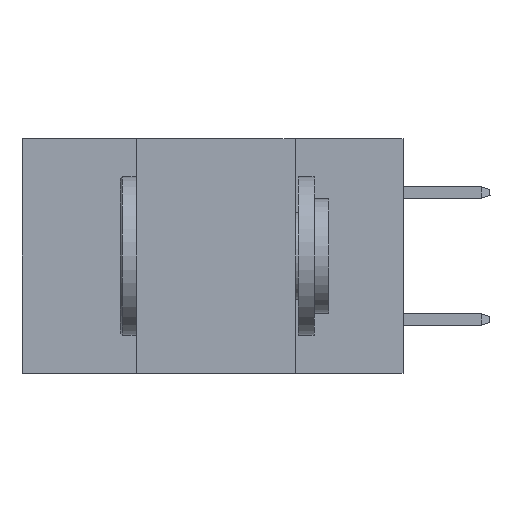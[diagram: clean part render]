
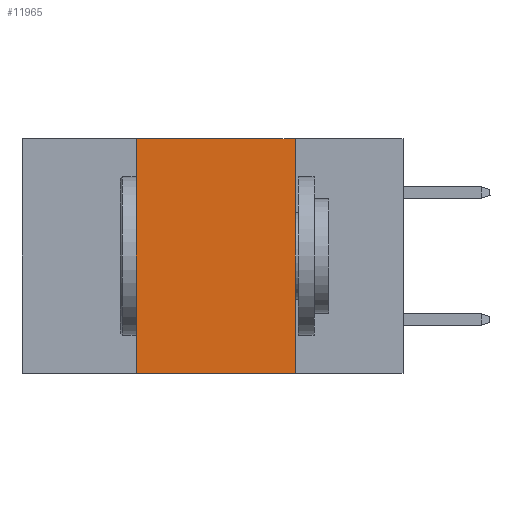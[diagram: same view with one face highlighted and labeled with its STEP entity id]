
A CAD part, left-side view. The second image highlights one B-rep face of the part: STEP entity #11965.
In plain terms, the highlighted planar face has unit normal (-1, 0, 0).
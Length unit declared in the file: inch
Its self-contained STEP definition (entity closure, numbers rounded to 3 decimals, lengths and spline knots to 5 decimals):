
#2201 = CARTESIAN_POINT ( 'NONE',  ( 0., 0.42, -0.37 ) ) ;
#2226 = CARTESIAN_POINT ( 'NONE',  ( 0., 0.6, 0. ) ) ;
#2872 = LINE ( 'NONE', #12746, #4598 ) ;
#4084 = LINE ( 'NONE', #10948, #7646 ) ;
#4598 = VECTOR ( 'NONE', #7721, 39.37008 ) ;
#5385 = DIRECTION ( 'NONE',  ( 0., 0., 1. ) ) ;
#5600 = VERTEX_POINT ( 'NONE', #17163 ) ;
#5842 = ORIENTED_EDGE ( 'NONE', *, *, #9859, .T. ) ;
#6105 = VECTOR ( 'NONE', #8890, 39.37008 ) ;
#6696 = VERTEX_POINT ( 'NONE', #13081 ) ;
#7169 = EDGE_LOOP ( 'NONE', ( #9057, #16360, #7323, #5842 ) ) ;
#7323 = ORIENTED_EDGE ( 'NONE', *, *, #16214, .F. ) ;
#7374 = DIRECTION ( 'NONE',  ( 0., -1., 0. ) ) ;
#7625 = DIRECTION ( 'NONE',  ( 0., 0., -1. ) ) ;
#7646 = VECTOR ( 'NONE', #7374, 39.37008 ) ;
#7721 = DIRECTION ( 'NONE',  ( 0., -1., 0. ) ) ;
#8514 = VERTEX_POINT ( 'NONE', #2201 ) ;
#8890 = DIRECTION ( 'NONE',  ( 0., 0., -1. ) ) ;
#9057 = ORIENTED_EDGE ( 'NONE', *, *, #13952, .F. ) ;
#9064 = VECTOR ( 'NONE', #5385, 39.37008 ) ;
#9099 = DIRECTION ( 'NONE',  ( 1., 0., 0. ) ) ;
#9204 = FACE_OUTER_BOUND ( 'NONE', #7169, .T. ) ;
#9859 = EDGE_CURVE ( 'NONE', #8514, #5600, #2872, .T. ) ;
#10443 = LINE ( 'NONE', #12225, #6105 ) ;
#10948 = CARTESIAN_POINT ( 'NONE',  ( 0., 0.6, 0. ) ) ;
#11965 = ADVANCED_FACE ( 'NONE', ( #9204 ), #17575, .F. ) ;
#12225 = CARTESIAN_POINT ( 'NONE',  ( 0., 0.17, 0. ) ) ;
#12746 = CARTESIAN_POINT ( 'NONE',  ( 0., 0.6, -0.37 ) ) ;
#13081 = CARTESIAN_POINT ( 'NONE',  ( 0., 0.17, 0. ) ) ;
#13438 = CARTESIAN_POINT ( 'NONE',  ( 0., 0.42, 0. ) ) ;
#13898 = LINE ( 'NONE', #16884, #9064 ) ;
#13952 = EDGE_CURVE ( 'NONE', #6696, #5600, #10443, .T. ) ;
#15003 = AXIS2_PLACEMENT_3D ( 'NONE', #2226, #9099, #7625 ) ;
#16214 = EDGE_CURVE ( 'NONE', #8514, #19929, #13898, .T. ) ;
#16360 = ORIENTED_EDGE ( 'NONE', *, *, #16676, .F. ) ;
#16676 = EDGE_CURVE ( 'NONE', #19929, #6696, #4084, .T. ) ;
#16884 = CARTESIAN_POINT ( 'NONE',  ( 0., 0.42, 0. ) ) ;
#17163 = CARTESIAN_POINT ( 'NONE',  ( 0., 0.17, -0.37 ) ) ;
#17575 = PLANE ( 'NONE',  #15003 ) ;
#19929 = VERTEX_POINT ( 'NONE', #13438 ) ;
